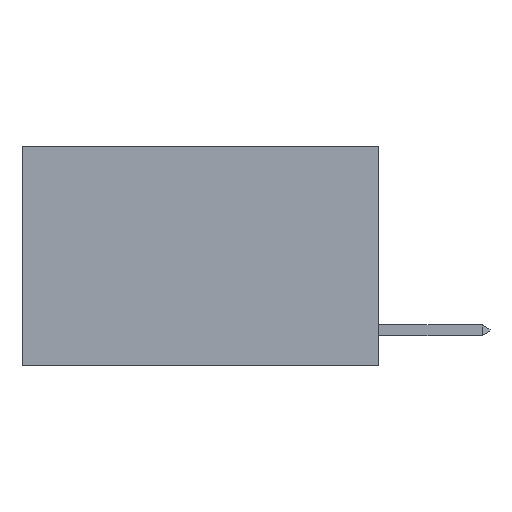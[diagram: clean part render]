
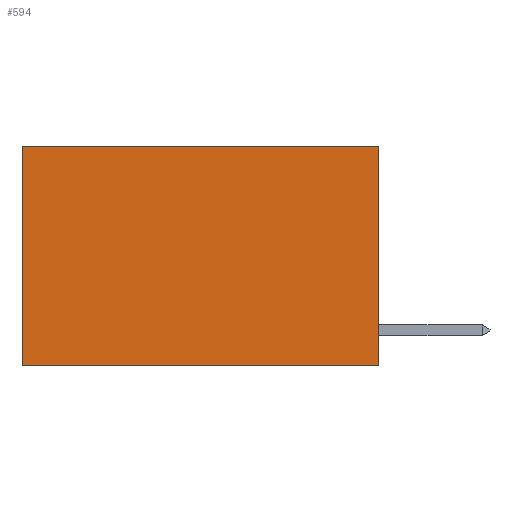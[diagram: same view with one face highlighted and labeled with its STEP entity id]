
A CAD part, left-side view. The second image highlights one B-rep face of the part: STEP entity #594.
In plain terms, the highlighted planar face has unit normal (-1, 0, 0).
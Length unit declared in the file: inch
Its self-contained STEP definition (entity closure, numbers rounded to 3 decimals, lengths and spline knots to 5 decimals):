
#97 = ORIENTED_EDGE ( 'NONE', *, *, #7066, .F. ) ;
#100 = CARTESIAN_POINT ( 'NONE',  ( 0.2625, 0.6, 0. ) ) ;
#111 = VECTOR ( 'NONE', #1934, 39.37008 ) ;
#594 = ADVANCED_FACE ( 'NONE', ( #8392 ), #8654, .F. ) ;
#634 = LINE ( 'NONE', #1743, #2326 ) ;
#655 = ORIENTED_EDGE ( 'NONE', *, *, #8395, .T. ) ;
#675 = VECTOR ( 'NONE', #9062, 39.37008 ) ;
#838 = VECTOR ( 'NONE', #6522, 39.37008 ) ;
#936 = LINE ( 'NONE', #6371, #838 ) ;
#1358 = DIRECTION ( 'NONE',  ( 0., 0., -1. ) ) ;
#1743 = CARTESIAN_POINT ( 'NONE',  ( 0.2625, 0., 0. ) ) ;
#1934 = DIRECTION ( 'NONE',  ( 0., 1., 0. ) ) ;
#2079 = EDGE_CURVE ( 'NONE', #9310, #4442, #936, .T. ) ;
#2127 = EDGE_LOOP ( 'NONE', ( #5877, #8094, #97, #655 ) ) ;
#2326 = VECTOR ( 'NONE', #2835, 39.37008 ) ;
#2543 = CARTESIAN_POINT ( 'NONE',  ( 0.2625, 0., 0. ) ) ;
#2736 = LINE ( 'NONE', #2543, #675 ) ;
#2793 = CARTESIAN_POINT ( 'NONE',  ( 0.2625, 0., 0. ) ) ;
#2835 = DIRECTION ( 'NONE',  ( 0., 0., -1. ) ) ;
#4075 = EDGE_CURVE ( 'NONE', #7715, #4442, #7010, .T. ) ;
#4224 = CARTESIAN_POINT ( 'NONE',  ( 0.2625, 0., 0. ) ) ;
#4356 = DIRECTION ( 'NONE',  ( 1., 0., 0. ) ) ;
#4442 = VERTEX_POINT ( 'NONE', #6256 ) ;
#4802 = CARTESIAN_POINT ( 'NONE',  ( 0.2625, 0., -0.37 ) ) ;
#5350 = VERTEX_POINT ( 'NONE', #4224 ) ;
#5877 = ORIENTED_EDGE ( 'NONE', *, *, #2079, .T. ) ;
#5993 = AXIS2_PLACEMENT_3D ( 'NONE', #2793, #4356, #1358 ) ;
#6256 = CARTESIAN_POINT ( 'NONE',  ( 0.2625, 0.6, -0.37 ) ) ;
#6371 = CARTESIAN_POINT ( 'NONE',  ( 0.2625, 0.6, 0. ) ) ;
#6522 = DIRECTION ( 'NONE',  ( 0., 0., -1. ) ) ;
#6540 = CARTESIAN_POINT ( 'NONE',  ( 0.2625, 0., -0.37 ) ) ;
#7010 = LINE ( 'NONE', #4802, #111 ) ;
#7066 = EDGE_CURVE ( 'NONE', #5350, #7715, #634, .T. ) ;
#7715 = VERTEX_POINT ( 'NONE', #6540 ) ;
#8094 = ORIENTED_EDGE ( 'NONE', *, *, #4075, .F. ) ;
#8392 = FACE_OUTER_BOUND ( 'NONE', #2127, .T. ) ;
#8395 = EDGE_CURVE ( 'NONE', #5350, #9310, #2736, .T. ) ;
#8654 = PLANE ( 'NONE',  #5993 ) ;
#9062 = DIRECTION ( 'NONE',  ( 0., 1., 0. ) ) ;
#9310 = VERTEX_POINT ( 'NONE', #100 ) ;
